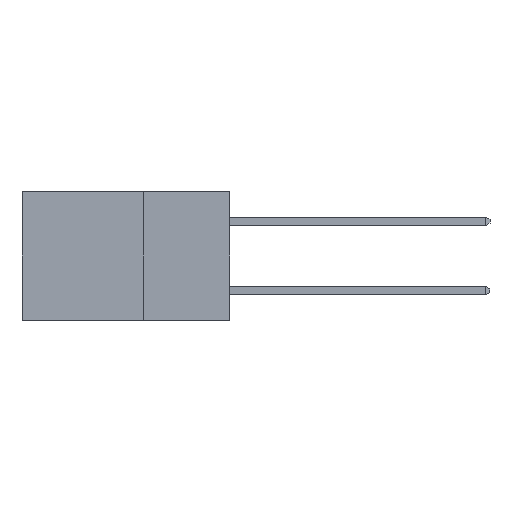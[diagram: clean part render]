
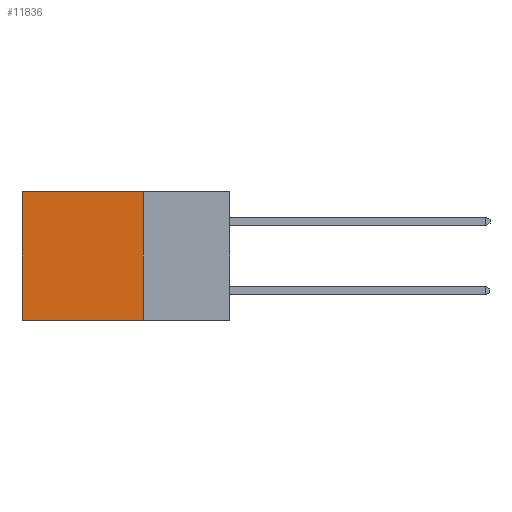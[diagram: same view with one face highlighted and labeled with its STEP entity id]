
A CAD part, left-side view. The second image highlights one B-rep face of the part: STEP entity #11836.
In plain terms, the highlighted planar face has unit normal (-1, 0, 0).
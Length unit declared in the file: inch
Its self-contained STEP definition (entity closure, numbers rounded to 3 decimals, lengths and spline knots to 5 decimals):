
#257 = CARTESIAN_POINT ( 'NONE',  ( 0.298, 0.6, -0.37 ) ) ;
#1006 = ORIENTED_EDGE ( 'NONE', *, *, #3255, .T. ) ;
#1044 = VERTEX_POINT ( 'NONE', #5237 ) ;
#1293 = CARTESIAN_POINT ( 'NONE',  ( 0.298, 0.6, 0. ) ) ;
#1403 = CARTESIAN_POINT ( 'NONE',  ( 0.298, 0.25, -0.37 ) ) ;
#1590 = PLANE ( 'NONE',  #10130 ) ;
#1749 = DIRECTION ( 'NONE',  ( 0., 1., 0. ) ) ;
#1751 = LINE ( 'NONE', #1895, #11342 ) ;
#1768 = VECTOR ( 'NONE', #9446, 39.37008 ) ;
#1895 = CARTESIAN_POINT ( 'NONE',  ( 0.298, 0.25, 0. ) ) ;
#2289 = LINE ( 'NONE', #1403, #4554 ) ;
#2350 = ORIENTED_EDGE ( 'NONE', *, *, #9287, .T. ) ;
#2897 = ORIENTED_EDGE ( 'NONE', *, *, #7870, .F. ) ;
#3255 = EDGE_CURVE ( 'NONE', #4328, #9599, #1751, .T. ) ;
#3439 = LINE ( 'NONE', #1293, #8053 ) ;
#3578 = CARTESIAN_POINT ( 'NONE',  ( 0.298, 0.25, 0. ) ) ;
#3670 = FACE_OUTER_BOUND ( 'NONE', #6086, .T. ) ;
#4328 = VERTEX_POINT ( 'NONE', #4486 ) ;
#4469 = DIRECTION ( 'NONE',  ( 0., 0., -1. ) ) ;
#4486 = CARTESIAN_POINT ( 'NONE',  ( 0.298, 0.25, 0. ) ) ;
#4554 = VECTOR ( 'NONE', #10720, 39.37008 ) ;
#5237 = CARTESIAN_POINT ( 'NONE',  ( 0.298, 0.25, -0.37 ) ) ;
#5767 = VERTEX_POINT ( 'NONE', #257 ) ;
#6057 = DIRECTION ( 'NONE',  ( 0., 0., -1. ) ) ;
#6086 = EDGE_LOOP ( 'NONE', ( #2350, #6812, #2897, #1006 ) ) ;
#6812 = ORIENTED_EDGE ( 'NONE', *, *, #10073, .F. ) ;
#7870 = EDGE_CURVE ( 'NONE', #4328, #1044, #11355, .T. ) ;
#8053 = VECTOR ( 'NONE', #6057, 39.37008 ) ;
#9287 = EDGE_CURVE ( 'NONE', #9599, #5767, #3439, .T. ) ;
#9446 = DIRECTION ( 'NONE',  ( 0., 0., -1. ) ) ;
#9599 = VERTEX_POINT ( 'NONE', #11823 ) ;
#10025 = DIRECTION ( 'NONE',  ( 1., 0., 0. ) ) ;
#10073 = EDGE_CURVE ( 'NONE', #1044, #5767, #2289, .T. ) ;
#10130 = AXIS2_PLACEMENT_3D ( 'NONE', #3578, #10025, #4469 ) ;
#10720 = DIRECTION ( 'NONE',  ( 0., 1., 0. ) ) ;
#11229 = CARTESIAN_POINT ( 'NONE',  ( 0.298, 0.25, 0. ) ) ;
#11342 = VECTOR ( 'NONE', #1749, 39.37008 ) ;
#11355 = LINE ( 'NONE', #11229, #1768 ) ;
#11823 = CARTESIAN_POINT ( 'NONE',  ( 0.298, 0.6, 0. ) ) ;
#11836 = ADVANCED_FACE ( 'NONE', ( #3670 ), #1590, .F. ) ;
